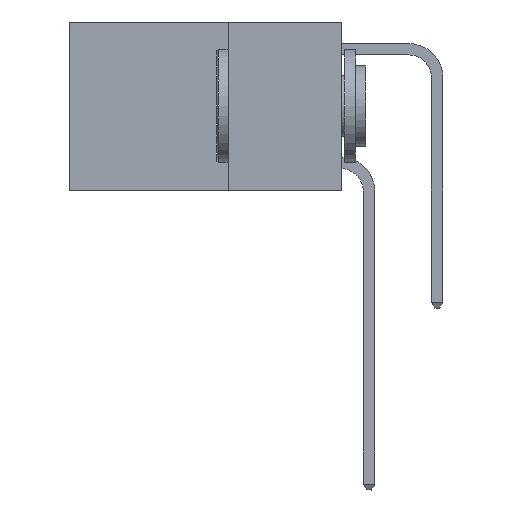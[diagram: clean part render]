
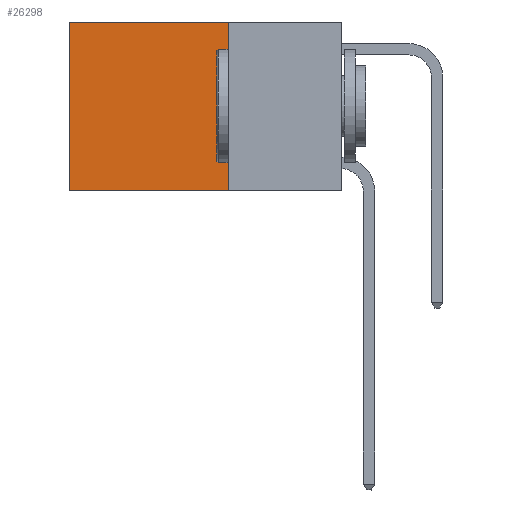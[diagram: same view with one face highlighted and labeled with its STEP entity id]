
A CAD part, left-side view. The second image highlights one B-rep face of the part: STEP entity #26298.
In plain terms, the highlighted planar face has unit normal (-1, 0, 0).
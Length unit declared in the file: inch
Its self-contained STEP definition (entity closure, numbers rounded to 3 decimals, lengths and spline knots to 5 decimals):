
#144 = VERTEX_POINT ( 'NONE', #17070 ) ;
#1235 = EDGE_CURVE ( 'NONE', #5720, #15121, #14904, .T. ) ;
#2102 = EDGE_LOOP ( 'NONE', ( #4094, #7052, #25948, #30708 ) ) ;
#2632 = CARTESIAN_POINT ( 'NONE',  ( 0.2625, 0.25, 0. ) ) ;
#3152 = EDGE_CURVE ( 'NONE', #5720, #144, #21058, .T. ) ;
#3273 = PLANE ( 'NONE',  #10357 ) ;
#4094 = ORIENTED_EDGE ( 'NONE', *, *, #6983, .T. ) ;
#5720 = VERTEX_POINT ( 'NONE', #30539 ) ;
#6416 = VERTEX_POINT ( 'NONE', #7447 ) ;
#6983 = EDGE_CURVE ( 'NONE', #144, #6416, #27113, .T. ) ;
#7052 = ORIENTED_EDGE ( 'NONE', *, *, #10826, .F. ) ;
#7272 = DIRECTION ( 'NONE',  ( 0., 1., 0. ) ) ;
#7447 = CARTESIAN_POINT ( 'NONE',  ( 0.2625, 0.6, -0.37 ) ) ;
#7994 = VECTOR ( 'NONE', #19741, 39.37008 ) ;
#8752 = DIRECTION ( 'NONE',  ( 0., 0., -1. ) ) ;
#9717 = CARTESIAN_POINT ( 'NONE',  ( 0.2625, 0.25, 0. ) ) ;
#10357 = AXIS2_PLACEMENT_3D ( 'NONE', #13752, #27318, #8752 ) ;
#10691 = DIRECTION ( 'NONE',  ( 0., 1., 0. ) ) ;
#10826 = EDGE_CURVE ( 'NONE', #15121, #6416, #23809, .T. ) ;
#11353 = VECTOR ( 'NONE', #7272, 39.37008 ) ;
#11470 = DIRECTION ( 'NONE',  ( 0., 0., -1. ) ) ;
#13752 = CARTESIAN_POINT ( 'NONE',  ( 0.2625, 0.25, 0. ) ) ;
#13919 = FACE_OUTER_BOUND ( 'NONE', #2102, .T. ) ;
#14904 = LINE ( 'NONE', #9717, #7994 ) ;
#15121 = VERTEX_POINT ( 'NONE', #18296 ) ;
#17070 = CARTESIAN_POINT ( 'NONE',  ( 0.2625, 0.6, 0. ) ) ;
#18296 = CARTESIAN_POINT ( 'NONE',  ( 0.2625, 0.25, -0.37 ) ) ;
#19741 = DIRECTION ( 'NONE',  ( 0., 0., -1. ) ) ;
#21058 = LINE ( 'NONE', #2632, #32183 ) ;
#23809 = LINE ( 'NONE', #26030, #11353 ) ;
#24568 = CARTESIAN_POINT ( 'NONE',  ( 0.2625, 0.6, 0. ) ) ;
#25948 = ORIENTED_EDGE ( 'NONE', *, *, #1235, .F. ) ;
#26030 = CARTESIAN_POINT ( 'NONE',  ( 0.2625, 0.25, -0.37 ) ) ;
#26298 = ADVANCED_FACE ( 'NONE', ( #13919 ), #3273, .F. ) ;
#27113 = LINE ( 'NONE', #24568, #27752 ) ;
#27318 = DIRECTION ( 'NONE',  ( 1., 0., 0. ) ) ;
#27752 = VECTOR ( 'NONE', #11470, 39.37008 ) ;
#30539 = CARTESIAN_POINT ( 'NONE',  ( 0.2625, 0.25, 0. ) ) ;
#30708 = ORIENTED_EDGE ( 'NONE', *, *, #3152, .T. ) ;
#32183 = VECTOR ( 'NONE', #10691, 39.37008 ) ;
